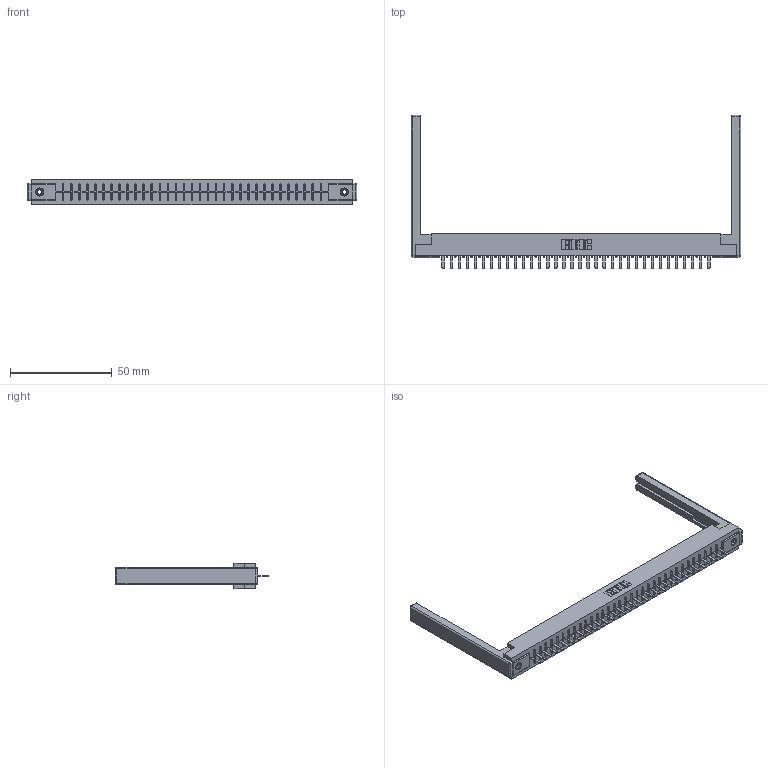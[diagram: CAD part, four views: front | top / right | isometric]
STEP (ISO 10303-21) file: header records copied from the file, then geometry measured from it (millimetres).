
FILE_DESCRIPTION (( 'STEP AP203' ), '1' );
FILE_NAME ('356-034-520-168.STEP', '2018-08-01T21:35:22', ( '' ), ( '' ), 'SwSTEP 2.0', 'SolidWorks 2016', '' );
FILE_SCHEMA (( 'CONFIG_CONTROL_DESIGN' ));
Length unit declared in the file: inch
Products named in the file (5): 345-250-001_345-250-001-102; 307-220-068; 356-034-520-168; 306 Part_.156 Dia; 306-290-001_120
Assembly tree (39 placements, depth 2):
  356-034-520-168
    306 Part_.156 Dia
    306-290-001_120  x34
    345-250-001_345-250-001-102  x2
    307-220-068  x2
Bounding box: 162.15 x 75.41 x 12.7 mm (x, y, z)
Volume: 22224.3 mm3; surface area: 22325.1 mm2
Topology: 39 solids, 39 shells, 2650 faces, 7404 edges, 4732 vertices
Faces by surface type: plane 1754, cylinder 736, sphere 144, cone 12, torus 4
Entity records: 35458 total; most frequent: CARTESIAN_POINT 5918, ORIENTED_EDGE 5858, DIRECTION 5849, EDGE_CURVE 2929, LINE 2283, VECTOR 2283, VERTEX_POINT 1852, AXIS2_PLACEMENT_3D 1783
